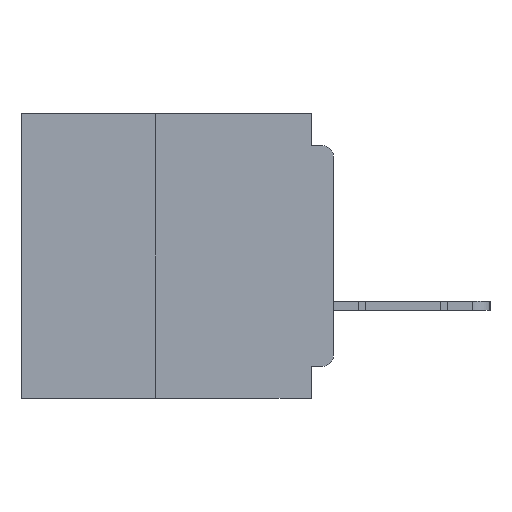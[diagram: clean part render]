
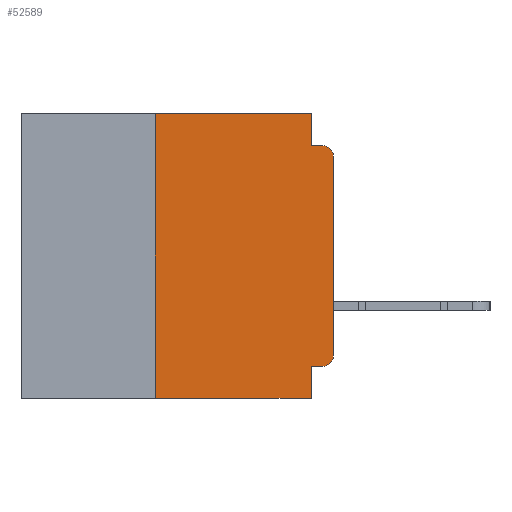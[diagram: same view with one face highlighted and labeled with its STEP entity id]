
A CAD part, left-side view. The second image highlights one B-rep face of the part: STEP entity #52589.
In plain terms, the highlighted planar face has unit normal (-1, 0, 0).
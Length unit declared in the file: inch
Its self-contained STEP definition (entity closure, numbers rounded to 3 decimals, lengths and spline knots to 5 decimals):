
#387 = CARTESIAN_POINT ( 'NONE',  ( 0., 0., -0.355 ) ) ;
#1138 = DIRECTION ( 'NONE',  ( -1., 0., 0. ) ) ;
#1766 = CARTESIAN_POINT ( 'NONE',  ( 0., 0.015, -0.34 ) ) ;
#2686 = ORIENTED_EDGE ( 'NONE', *, *, #42553, .F. ) ;
#3097 = VECTOR ( 'NONE', #56413, 39.37008 ) ;
#3811 = CARTESIAN_POINT ( 'NONE',  ( 0., 0.437, 0. ) ) ;
#4631 = VERTEX_POINT ( 'NONE', #55530 ) ;
#5285 = ORIENTED_EDGE ( 'NONE', *, *, #7963, .T. ) ;
#7035 = DIRECTION ( 'NONE',  ( 0., 0., -1. ) ) ;
#7963 = EDGE_CURVE ( 'NONE', #20157, #4631, #44923, .T. ) ;
#9100 = DIRECTION ( 'NONE',  ( 1., 0., 0. ) ) ;
#9926 = EDGE_CURVE ( 'NONE', #51575, #11013, #36533, .T. ) ;
#10418 = CARTESIAN_POINT ( 'NONE',  ( 0., 0.25, 0. ) ) ;
#11006 = EDGE_CURVE ( 'NONE', #11013, #16156, #41386, .T. ) ;
#11013 = VERTEX_POINT ( 'NONE', #25118 ) ;
#12797 = VERTEX_POINT ( 'NONE', #33443 ) ;
#16156 = VERTEX_POINT ( 'NONE', #23153 ) ;
#16821 = ORIENTED_EDGE ( 'NONE', *, *, #56117, .F. ) ;
#20157 = VERTEX_POINT ( 'NONE', #56492 ) ;
#20301 = DIRECTION ( 'NONE',  ( 0., 0., 1. ) ) ;
#20710 = ORIENTED_EDGE ( 'NONE', *, *, #11006, .F. ) ;
#22783 = VECTOR ( 'NONE', #57702, 39.37008 ) ;
#23153 = CARTESIAN_POINT ( 'NONE',  ( 0., 0.031, -0.4 ) ) ;
#24642 = CARTESIAN_POINT ( 'NONE',  ( 0., 0.031, 0. ) ) ;
#25118 = CARTESIAN_POINT ( 'NONE',  ( 0., 0.031, -0.355 ) ) ;
#25189 = DIRECTION ( 'NONE',  ( 0., -1., 0. ) ) ;
#26795 = VERTEX_POINT ( 'NONE', #34831 ) ;
#27081 = AXIS2_PLACEMENT_3D ( 'NONE', #1766, #38176, #7035 ) ;
#27778 = VECTOR ( 'NONE', #64875, 39.37008 ) ;
#29152 = DIRECTION ( 'NONE',  ( 0., 0., 1. ) ) ;
#32340 = CARTESIAN_POINT ( 'NONE',  ( 0., 0.015, -0.06 ) ) ;
#32663 = VECTOR ( 'NONE', #29152, 39.37008 ) ;
#32770 = ORIENTED_EDGE ( 'NONE', *, *, #44413, .F. ) ;
#33443 = CARTESIAN_POINT ( 'NONE',  ( 0., 0.031, 0. ) ) ;
#34513 = ORIENTED_EDGE ( 'NONE', *, *, #42035, .F. ) ;
#34831 = CARTESIAN_POINT ( 'NONE',  ( 0., 0.25, -0.4 ) ) ;
#34999 = PLANE ( 'NONE',  #46806 ) ;
#35066 = DIRECTION ( 'NONE',  ( 0., 0., -1. ) ) ;
#36533 = LINE ( 'NONE', #387, #22783 ) ;
#36731 = CARTESIAN_POINT ( 'NONE',  ( 0., 0.015, -0.355 ) ) ;
#37559 = DIRECTION ( 'NONE',  ( 0., 0., -1. ) ) ;
#38176 = DIRECTION ( 'NONE',  ( -1., 0., 0. ) ) ;
#39043 = CARTESIAN_POINT ( 'NONE',  ( 0., 0., -0.045 ) ) ;
#40327 = FACE_OUTER_BOUND ( 'NONE', #43440, .T. ) ;
#41386 = LINE ( 'NONE', #51221, #3097 ) ;
#42035 = EDGE_CURVE ( 'NONE', #26795, #49334, #46522, .T. ) ;
#42553 = EDGE_CURVE ( 'NONE', #66478, #4631, #55317, .T. ) ;
#43059 = CARTESIAN_POINT ( 'NONE',  ( 0., 0.031, -0.045 ) ) ;
#43440 = EDGE_LOOP ( 'NONE', ( #54895, #5285, #2686, #32770, #16821, #34513, #62868, #20710, #67324, #55806 ) ) ;
#44413 = EDGE_CURVE ( 'NONE', #12797, #66478, #67265, .T. ) ;
#44923 = CIRCLE ( 'NONE', #51768, 0.015 ) ;
#45463 = DIRECTION ( 'NONE',  ( 0., 0., -1. ) ) ;
#46192 = CARTESIAN_POINT ( 'NONE',  ( 0., 0., 0. ) ) ;
#46522 = LINE ( 'NONE', #54995, #32663 ) ;
#46806 = AXIS2_PLACEMENT_3D ( 'NONE', #3811, #9100, #45463 ) ;
#47491 = EDGE_CURVE ( 'NONE', #55103, #20157, #51700, .T. ) ;
#47581 = CARTESIAN_POINT ( 'NONE',  ( 0., 0., -0.34 ) ) ;
#47809 = CARTESIAN_POINT ( 'NONE',  ( 0., 0.437, -0.4 ) ) ;
#49334 = VERTEX_POINT ( 'NONE', #10418 ) ;
#50246 = VECTOR ( 'NONE', #52967, 39.37008 ) ;
#51221 = CARTESIAN_POINT ( 'NONE',  ( 0., 0.031, -0.4 ) ) ;
#51295 = LINE ( 'NONE', #66419, #61792 ) ;
#51575 = VERTEX_POINT ( 'NONE', #36731 ) ;
#51700 = LINE ( 'NONE', #46192, #65431 ) ;
#51768 = AXIS2_PLACEMENT_3D ( 'NONE', #32340, #1138, #37559 ) ;
#52589 = ADVANCED_FACE ( 'NONE', ( #40327 ), #34999, .F. ) ;
#52967 = DIRECTION ( 'NONE',  ( 0., -1., 0. ) ) ;
#53512 = VECTOR ( 'NONE', #35066, 39.37008 ) ;
#54895 = ORIENTED_EDGE ( 'NONE', *, *, #47491, .T. ) ;
#54995 = CARTESIAN_POINT ( 'NONE',  ( 0., 0.25, -0.4 ) ) ;
#55103 = VERTEX_POINT ( 'NONE', #47581 ) ;
#55317 = LINE ( 'NONE', #39043, #27778 ) ;
#55530 = CARTESIAN_POINT ( 'NONE',  ( 0., 0.015, -0.045 ) ) ;
#55806 = ORIENTED_EDGE ( 'NONE', *, *, #58915, .T. ) ;
#56117 = EDGE_CURVE ( 'NONE', #49334, #12797, #51295, .T. ) ;
#56413 = DIRECTION ( 'NONE',  ( 0., 0., -1. ) ) ;
#56492 = CARTESIAN_POINT ( 'NONE',  ( 0., 0., -0.06 ) ) ;
#57702 = DIRECTION ( 'NONE',  ( 0., 1., 0. ) ) ;
#58915 = EDGE_CURVE ( 'NONE', #51575, #55103, #64377, .T. ) ;
#61792 = VECTOR ( 'NONE', #25189, 39.37008 ) ;
#62352 = LINE ( 'NONE', #47809, #50246 ) ;
#62868 = ORIENTED_EDGE ( 'NONE', *, *, #63357, .T. ) ;
#63357 = EDGE_CURVE ( 'NONE', #26795, #16156, #62352, .T. ) ;
#64377 = CIRCLE ( 'NONE', #27081, 0.015 ) ;
#64875 = DIRECTION ( 'NONE',  ( 0., -1., 0. ) ) ;
#65431 = VECTOR ( 'NONE', #20301, 39.37008 ) ;
#66419 = CARTESIAN_POINT ( 'NONE',  ( 0., 0.437, 0. ) ) ;
#66478 = VERTEX_POINT ( 'NONE', #43059 ) ;
#67265 = LINE ( 'NONE', #24642, #53512 ) ;
#67324 = ORIENTED_EDGE ( 'NONE', *, *, #9926, .F. ) ;
